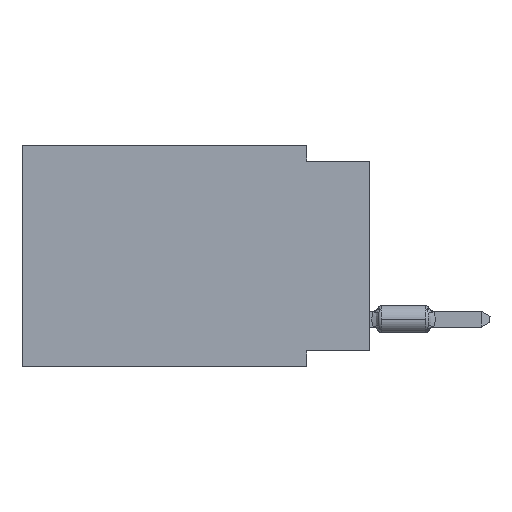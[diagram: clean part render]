
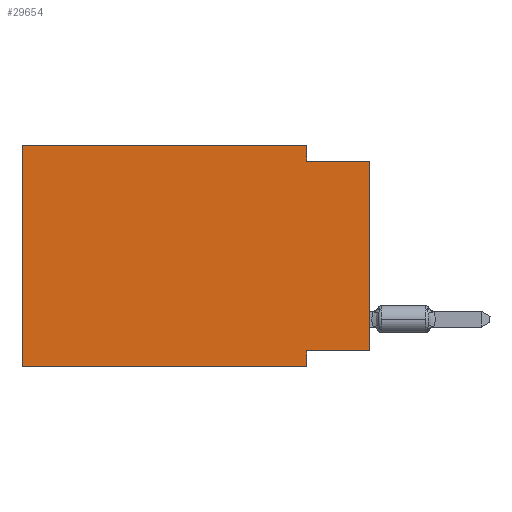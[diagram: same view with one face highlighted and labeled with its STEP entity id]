
A CAD part, left-side view. The second image highlights one B-rep face of the part: STEP entity #29654.
In plain terms, the highlighted planar face has unit normal (-1, 0, 0).
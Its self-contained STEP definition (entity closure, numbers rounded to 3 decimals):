
#811 = LINE ( 'NONE', #10658, #11898 ) ;
#819 = VECTOR ( 'NONE', #28927, 1000. ) ;
#1009 = DIRECTION ( 'NONE',  ( 0., 1., 0. ) ) ;
#1141 = LINE ( 'NONE', #25470, #15548 ) ;
#2053 = CARTESIAN_POINT ( 'NONE',  ( 0., 0., -8.255 ) ) ;
#2179 = CARTESIAN_POINT ( 'NONE',  ( 0., 2.54, -8.89 ) ) ;
#2221 = VECTOR ( 'NONE', #29783, 1000. ) ;
#2299 = CARTESIAN_POINT ( 'NONE',  ( 0., 0., -0.635 ) ) ;
#2991 = CARTESIAN_POINT ( 'NONE',  ( 0., 13.97, 0. ) ) ;
#3120 = FACE_OUTER_BOUND ( 'NONE', #24605, .T. ) ;
#4972 = VERTEX_POINT ( 'NONE', #15140 ) ;
#4997 = CARTESIAN_POINT ( 'NONE',  ( 0., 13.97, -8.89 ) ) ;
#5182 = CARTESIAN_POINT ( 'NONE',  ( 0., 2.54, 0. ) ) ;
#6436 = VECTOR ( 'NONE', #18560, 1000. ) ;
#6778 = VECTOR ( 'NONE', #29027, 1000. ) ;
#7430 = LINE ( 'NONE', #2179, #819 ) ;
#8265 = DIRECTION ( 'NONE',  ( 0., -1., 0. ) ) ;
#8387 = VECTOR ( 'NONE', #1009, 1000. ) ;
#8501 = VERTEX_POINT ( 'NONE', #28930 ) ;
#8859 = DIRECTION ( 'NONE',  ( 0., -1., 0. ) ) ;
#9143 = LINE ( 'NONE', #2299, #6778 ) ;
#9781 = DIRECTION ( 'NONE',  ( 0., 0., -1. ) ) ;
#10395 = ORIENTED_EDGE ( 'NONE', *, *, #22132, .F. ) ;
#10658 = CARTESIAN_POINT ( 'NONE',  ( 0., 13.97, -8.89 ) ) ;
#10742 = CARTESIAN_POINT ( 'NONE',  ( 0., 0., -0.635 ) ) ;
#11898 = VECTOR ( 'NONE', #8859, 1000. ) ;
#12685 = ORIENTED_EDGE ( 'NONE', *, *, #30598, .F. ) ;
#13060 = CARTESIAN_POINT ( 'NONE',  ( 0., 2.54, 0. ) ) ;
#14189 = CARTESIAN_POINT ( 'NONE',  ( 0., 2.54, -8.89 ) ) ;
#15044 = CARTESIAN_POINT ( 'NONE',  ( 0., 13.97, 0. ) ) ;
#15140 = CARTESIAN_POINT ( 'NONE',  ( 0., 2.54, -8.255 ) ) ;
#15548 = VECTOR ( 'NONE', #20847, 1000. ) ;
#15592 = LINE ( 'NONE', #25890, #17480 ) ;
#16369 = ORIENTED_EDGE ( 'NONE', *, *, #29877, .F. ) ;
#16596 = VERTEX_POINT ( 'NONE', #2991 ) ;
#17374 = VERTEX_POINT ( 'NONE', #2053 ) ;
#17414 = PLANE ( 'NONE',  #21500 ) ;
#17480 = VECTOR ( 'NONE', #8265, 1000. ) ;
#18347 = VERTEX_POINT ( 'NONE', #4997 ) ;
#18560 = DIRECTION ( 'NONE',  ( 0., 0., 1. ) ) ;
#18667 = VERTEX_POINT ( 'NONE', #14189 ) ;
#18929 = EDGE_CURVE ( 'NONE', #16596, #19239, #15592, .T. ) ;
#18931 = EDGE_CURVE ( 'NONE', #18347, #18667, #811, .T. ) ;
#19009 = ORIENTED_EDGE ( 'NONE', *, *, #23400, .F. ) ;
#19239 = VERTEX_POINT ( 'NONE', #5182 ) ;
#19933 = ORIENTED_EDGE ( 'NONE', *, *, #18929, .F. ) ;
#20245 = CARTESIAN_POINT ( 'NONE',  ( 0., 0., -8.255 ) ) ;
#20623 = ORIENTED_EDGE ( 'NONE', *, *, #21086, .F. ) ;
#20847 = DIRECTION ( 'NONE',  ( 0., 0., 1. ) ) ;
#21086 = EDGE_CURVE ( 'NONE', #17374, #4972, #22797, .T. ) ;
#21500 = AXIS2_PLACEMENT_3D ( 'NONE', #15044, #24753, #9781 ) ;
#22132 = EDGE_CURVE ( 'NONE', #18347, #16596, #30365, .T. ) ;
#22144 = ORIENTED_EDGE ( 'NONE', *, *, #18931, .T. ) ;
#22797 = LINE ( 'NONE', #20245, #8387 ) ;
#23400 = EDGE_CURVE ( 'NONE', #4972, #18667, #7430, .T. ) ;
#23524 = ORIENTED_EDGE ( 'NONE', *, *, #25391, .T. ) ;
#23761 = VERTEX_POINT ( 'NONE', #10742 ) ;
#24605 = EDGE_LOOP ( 'NONE', ( #23524, #16369, #12685, #19933, #10395, #22144, #19009, #20623 ) ) ;
#24753 = DIRECTION ( 'NONE',  ( 1., 0., 0. ) ) ;
#25391 = EDGE_CURVE ( 'NONE', #17374, #23761, #1141, .T. ) ;
#25470 = CARTESIAN_POINT ( 'NONE',  ( 0., 0., 0. ) ) ;
#25566 = CARTESIAN_POINT ( 'NONE',  ( 0., 13.97, 0. ) ) ;
#25890 = CARTESIAN_POINT ( 'NONE',  ( 0., 13.97, 0. ) ) ;
#28927 = DIRECTION ( 'NONE',  ( 0., 0., -1. ) ) ;
#28930 = CARTESIAN_POINT ( 'NONE',  ( 0., 2.54, -0.635 ) ) ;
#29027 = DIRECTION ( 'NONE',  ( 0., -1., 0. ) ) ;
#29654 = ADVANCED_FACE ( 'NONE', ( #3120 ), #17414, .F. ) ;
#29783 = DIRECTION ( 'NONE',  ( 0., 0., -1. ) ) ;
#29877 = EDGE_CURVE ( 'NONE', #8501, #23761, #9143, .T. ) ;
#30084 = LINE ( 'NONE', #13060, #2221 ) ;
#30365 = LINE ( 'NONE', #25566, #6436 ) ;
#30598 = EDGE_CURVE ( 'NONE', #19239, #8501, #30084, .T. ) ;
